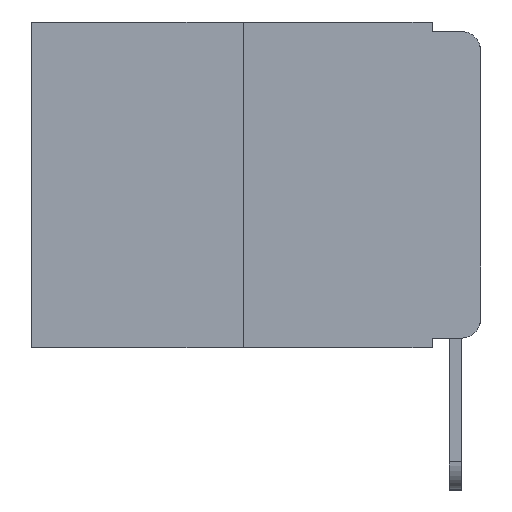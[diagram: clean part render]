
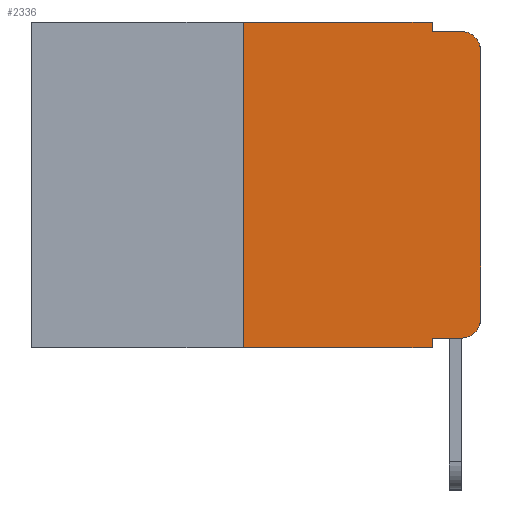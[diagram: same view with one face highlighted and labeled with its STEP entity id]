
A CAD part, left-side view. The second image highlights one B-rep face of the part: STEP entity #2336.
In plain terms, the highlighted planar face has unit normal (-1, 0, 0).
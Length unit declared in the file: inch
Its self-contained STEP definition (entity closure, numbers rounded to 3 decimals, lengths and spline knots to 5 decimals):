
#230 = VERTEX_POINT ( 'NONE', #15128 ) ;
#307 = VECTOR ( 'NONE', #9125, 39.37008 ) ;
#1818 = ORIENTED_EDGE ( 'NONE', *, *, #7007, .F. ) ;
#1872 = CARTESIAN_POINT ( 'NONE',  ( 0., 0.25, 0. ) ) ;
#2006 = EDGE_LOOP ( 'NONE', ( #4810, #12897, #17062, #1818, #14236, #7909, #15574, #4553, #8888, #13135 ) ) ;
#2336 = ADVANCED_FACE ( 'NONE', ( #11247 ), #12982, .F. ) ;
#2460 = CARTESIAN_POINT ( 'NONE',  ( 0., 0.051, -0.333 ) ) ;
#2689 = CARTESIAN_POINT ( 'NONE',  ( 0., 0.02, -0.03 ) ) ;
#2764 = CARTESIAN_POINT ( 'NONE',  ( 0., 0., 0. ) ) ;
#2779 = VERTEX_POINT ( 'NONE', #2460 ) ;
#2847 = CARTESIAN_POINT ( 'NONE',  ( 0., 0.051, -0.333 ) ) ;
#3256 = VERTEX_POINT ( 'NONE', #10707 ) ;
#3727 = VECTOR ( 'NONE', #4566, 39.37008 ) ;
#3775 = DIRECTION ( 'NONE',  ( 1., 0., 0. ) ) ;
#4359 = VERTEX_POINT ( 'NONE', #6175 ) ;
#4418 = DIRECTION ( 'NONE',  ( 0., 0., -1. ) ) ;
#4490 = CARTESIAN_POINT ( 'NONE',  ( 0., 0.02, -0.313 ) ) ;
#4553 = ORIENTED_EDGE ( 'NONE', *, *, #6911, .F. ) ;
#4566 = DIRECTION ( 'NONE',  ( 0., -1., 0. ) ) ;
#4810 = ORIENTED_EDGE ( 'NONE', *, *, #7058, .T. ) ;
#4901 = VERTEX_POINT ( 'NONE', #10947 ) ;
#4916 = AXIS2_PLACEMENT_3D ( 'NONE', #4490, #15012, #6192 ) ;
#5043 = CIRCLE ( 'NONE', #12102, 0.02 ) ;
#6061 = EDGE_CURVE ( 'NONE', #14911, #17322, #15790, .T. ) ;
#6175 = CARTESIAN_POINT ( 'NONE',  ( 0., 0.25, -0.343 ) ) ;
#6192 = DIRECTION ( 'NONE',  ( 0., 0., -1. ) ) ;
#6888 = EDGE_CURVE ( 'NONE', #230, #3256, #16210, .T. ) ;
#6910 = EDGE_CURVE ( 'NONE', #2779, #230, #8138, .T. ) ;
#6911 = EDGE_CURVE ( 'NONE', #2779, #13550, #15773, .T. ) ;
#6972 = EDGE_CURVE ( 'NONE', #4359, #13550, #10662, .T. ) ;
#7004 = EDGE_CURVE ( 'NONE', #4359, #14911, #9334, .T. ) ;
#7007 = EDGE_CURVE ( 'NONE', #17322, #4901, #16841, .T. ) ;
#7028 = EDGE_CURVE ( 'NONE', #4901, #17933, #8863, .T. ) ;
#7031 = EDGE_CURVE ( 'NONE', #19371, #17933, #5043, .T. ) ;
#7058 = EDGE_CURVE ( 'NONE', #3256, #19371, #19599, .T. ) ;
#7457 = CARTESIAN_POINT ( 'NONE',  ( 0., 0.473, -0.343 ) ) ;
#7666 = DIRECTION ( 'NONE',  ( 0., -1., 0. ) ) ;
#7874 = VECTOR ( 'NONE', #13604, 39.37008 ) ;
#7909 = ORIENTED_EDGE ( 'NONE', *, *, #7004, .F. ) ;
#8138 = LINE ( 'NONE', #2847, #3727 ) ;
#8277 = CARTESIAN_POINT ( 'NONE',  ( 0., 0., -0.03 ) ) ;
#8863 = LINE ( 'NONE', #17682, #15982 ) ;
#8888 = ORIENTED_EDGE ( 'NONE', *, *, #6910, .T. ) ;
#9125 = DIRECTION ( 'NONE',  ( 0., 0., 1. ) ) ;
#9334 = LINE ( 'NONE', #16249, #307 ) ;
#9646 = CARTESIAN_POINT ( 'NONE',  ( 0., 0.473, 0. ) ) ;
#9726 = CARTESIAN_POINT ( 'NONE',  ( 0., 0.051, 0. ) ) ;
#10662 = LINE ( 'NONE', #7457, #14007 ) ;
#10707 = CARTESIAN_POINT ( 'NONE',  ( 0., 0., -0.313 ) ) ;
#10743 = CARTESIAN_POINT ( 'NONE',  ( 0., 0.051, -0.343 ) ) ;
#10947 = CARTESIAN_POINT ( 'NONE',  ( 0., 0.051, -0.01 ) ) ;
#11247 = FACE_OUTER_BOUND ( 'NONE', #2006, .T. ) ;
#11548 = VECTOR ( 'NONE', #16487, 39.37008 ) ;
#12022 = CARTESIAN_POINT ( 'NONE',  ( 0., 0.02, -0.01 ) ) ;
#12049 = CARTESIAN_POINT ( 'NONE',  ( 0., 0.051, 0. ) ) ;
#12102 = AXIS2_PLACEMENT_3D ( 'NONE', #2689, #13543, #4418 ) ;
#12667 = VECTOR ( 'NONE', #13481, 39.37008 ) ;
#12897 = ORIENTED_EDGE ( 'NONE', *, *, #7031, .T. ) ;
#12982 = PLANE ( 'NONE',  #18471 ) ;
#13135 = ORIENTED_EDGE ( 'NONE', *, *, #6888, .T. ) ;
#13357 = DIRECTION ( 'NONE',  ( 0., -1., 0. ) ) ;
#13481 = DIRECTION ( 'NONE',  ( 0., 0., -1. ) ) ;
#13543 = DIRECTION ( 'NONE',  ( -1., 0., 0. ) ) ;
#13550 = VERTEX_POINT ( 'NONE', #10743 ) ;
#13604 = DIRECTION ( 'NONE',  ( 0., 0., 1. ) ) ;
#13940 = DIRECTION ( 'NONE',  ( 0., -1., 0. ) ) ;
#14007 = VECTOR ( 'NONE', #13357, 39.37008 ) ;
#14236 = ORIENTED_EDGE ( 'NONE', *, *, #6061, .F. ) ;
#14350 = CARTESIAN_POINT ( 'NONE',  ( 0., 0.473, 0. ) ) ;
#14406 = DIRECTION ( 'NONE',  ( 0., 0., -1. ) ) ;
#14911 = VERTEX_POINT ( 'NONE', #1872 ) ;
#15012 = DIRECTION ( 'NONE',  ( -1., 0., 0. ) ) ;
#15071 = CARTESIAN_POINT ( 'NONE',  ( 0., 0.051, 0. ) ) ;
#15128 = CARTESIAN_POINT ( 'NONE',  ( 0., 0.02, -0.333 ) ) ;
#15574 = ORIENTED_EDGE ( 'NONE', *, *, #6972, .T. ) ;
#15773 = LINE ( 'NONE', #15071, #11548 ) ;
#15790 = LINE ( 'NONE', #9646, #19002 ) ;
#15982 = VECTOR ( 'NONE', #7666, 39.37008 ) ;
#16210 = CIRCLE ( 'NONE', #4916, 0.02 ) ;
#16249 = CARTESIAN_POINT ( 'NONE',  ( 0., 0.25, 0. ) ) ;
#16487 = DIRECTION ( 'NONE',  ( 0., 0., -1. ) ) ;
#16841 = LINE ( 'NONE', #12049, #12667 ) ;
#17062 = ORIENTED_EDGE ( 'NONE', *, *, #7028, .F. ) ;
#17322 = VERTEX_POINT ( 'NONE', #9726 ) ;
#17682 = CARTESIAN_POINT ( 'NONE',  ( 0., 0.051, -0.01 ) ) ;
#17933 = VERTEX_POINT ( 'NONE', #12022 ) ;
#18471 = AXIS2_PLACEMENT_3D ( 'NONE', #14350, #3775, #14406 ) ;
#19002 = VECTOR ( 'NONE', #13940, 39.37008 ) ;
#19371 = VERTEX_POINT ( 'NONE', #8277 ) ;
#19599 = LINE ( 'NONE', #2764, #7874 ) ;
